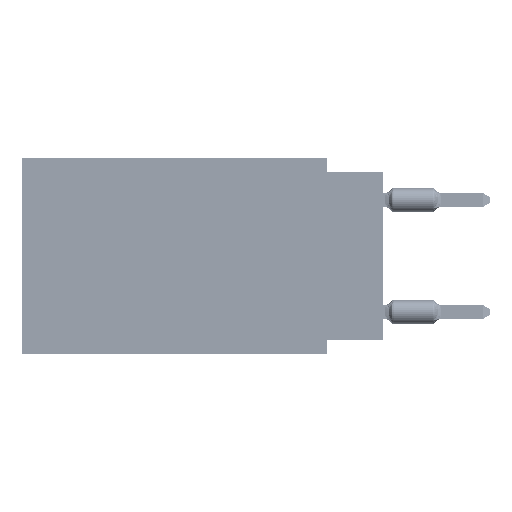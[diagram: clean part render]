
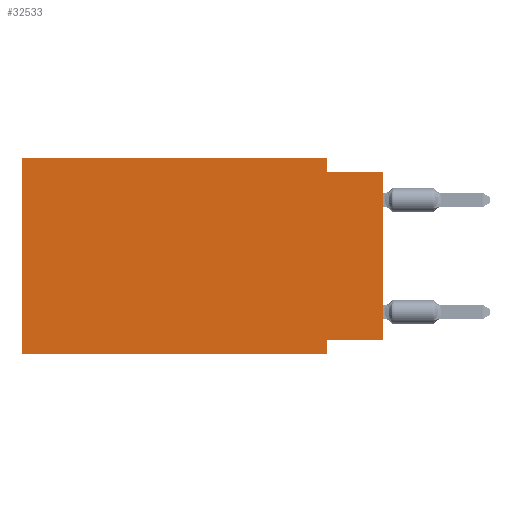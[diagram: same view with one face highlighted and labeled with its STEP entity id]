
A CAD part, left-side view. The second image highlights one B-rep face of the part: STEP entity #32533.
In plain terms, the highlighted planar face has unit normal (-1, 0, 0).
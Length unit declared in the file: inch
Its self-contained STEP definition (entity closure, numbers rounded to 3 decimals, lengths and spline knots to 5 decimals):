
#1469 = CARTESIAN_POINT ( 'NONE',  ( 0., 0., -0.025 ) ) ;
#1989 = EDGE_CURVE ( 'NONE', #17932, #36386, #73937, .T. ) ;
#2767 = CARTESIAN_POINT ( 'NONE',  ( 0., 0., -0.325 ) ) ;
#3506 = VERTEX_POINT ( 'NONE', #106104 ) ;
#4464 = DIRECTION ( 'NONE',  ( 0., 0., 1. ) ) ;
#6287 = ORIENTED_EDGE ( 'NONE', *, *, #96938, .T. ) ;
#7611 = CARTESIAN_POINT ( 'NONE',  ( 0., 0.1, -0.35 ) ) ;
#8929 = DIRECTION ( 'NONE',  ( 0., 0., -1. ) ) ;
#13136 = ORIENTED_EDGE ( 'NONE', *, *, #74413, .F. ) ;
#14028 = ORIENTED_EDGE ( 'NONE', *, *, #56712, .T. ) ;
#16276 = DIRECTION ( 'NONE',  ( 0., -1., 0. ) ) ;
#16744 = VECTOR ( 'NONE', #32953, 39.37008 ) ;
#17932 = VERTEX_POINT ( 'NONE', #60454 ) ;
#20745 = CARTESIAN_POINT ( 'NONE',  ( 0., 0., 0. ) ) ;
#21174 = CARTESIAN_POINT ( 'NONE',  ( 0., 0., -0.025 ) ) ;
#21676 = VERTEX_POINT ( 'NONE', #71001 ) ;
#21886 = DIRECTION ( 'NONE',  ( 0., 0., -1. ) ) ;
#26536 = VECTOR ( 'NONE', #16276, 39.37008 ) ;
#27663 = CARTESIAN_POINT ( 'NONE',  ( 0., 0.645, 0. ) ) ;
#29261 = LINE ( 'NONE', #21174, #70019 ) ;
#31399 = VERTEX_POINT ( 'NONE', #34176 ) ;
#32533 = ADVANCED_FACE ( 'NONE', ( #81167 ), #87672, .F. ) ;
#32953 = DIRECTION ( 'NONE',  ( 0., 0., -1. ) ) ;
#32995 = ORIENTED_EDGE ( 'NONE', *, *, #41083, .F. ) ;
#33418 = AXIS2_PLACEMENT_3D ( 'NONE', #56347, #55303, #21886 ) ;
#33515 = CARTESIAN_POINT ( 'NONE',  ( 0., 0.645, -0.35 ) ) ;
#34176 = CARTESIAN_POINT ( 'NONE',  ( 0., 0., -0.325 ) ) ;
#36386 = VERTEX_POINT ( 'NONE', #44296 ) ;
#36723 = LINE ( 'NONE', #2767, #80894 ) ;
#39363 = CARTESIAN_POINT ( 'NONE',  ( 0., 0.1, -0.025 ) ) ;
#40755 = CARTESIAN_POINT ( 'NONE',  ( 0., 0.1, 0. ) ) ;
#41083 = EDGE_CURVE ( 'NONE', #31399, #17932, #36723, .T. ) ;
#44296 = CARTESIAN_POINT ( 'NONE',  ( 0., 0.1, -0.35 ) ) ;
#44341 = LINE ( 'NONE', #27663, #56778 ) ;
#45364 = VECTOR ( 'NONE', #8929, 39.37008 ) ;
#49204 = LINE ( 'NONE', #82639, #53402 ) ;
#51661 = CARTESIAN_POINT ( 'NONE',  ( 0., 0.645, -0.35 ) ) ;
#51704 = VERTEX_POINT ( 'NONE', #39363 ) ;
#53402 = VECTOR ( 'NONE', #74020, 39.37008 ) ;
#53486 = VERTEX_POINT ( 'NONE', #1469 ) ;
#54056 = DIRECTION ( 'NONE',  ( 0., -1., 0. ) ) ;
#55303 = DIRECTION ( 'NONE',  ( 1., 0., 0. ) ) ;
#56347 = CARTESIAN_POINT ( 'NONE',  ( 0., 0.645, 0. ) ) ;
#56411 = LINE ( 'NONE', #40755, #45364 ) ;
#56712 = EDGE_CURVE ( 'NONE', #60900, #36386, #75028, .T. ) ;
#56778 = VECTOR ( 'NONE', #4464, 39.37008 ) ;
#60115 = EDGE_CURVE ( 'NONE', #51704, #53486, #29261, .T. ) ;
#60454 = CARTESIAN_POINT ( 'NONE',  ( 0., 0.1, -0.325 ) ) ;
#60900 = VERTEX_POINT ( 'NONE', #51661 ) ;
#67042 = ORIENTED_EDGE ( 'NONE', *, *, #84600, .F. ) ;
#70019 = VECTOR ( 'NONE', #54056, 39.37008 ) ;
#71001 = CARTESIAN_POINT ( 'NONE',  ( 0., 0.1, 0. ) ) ;
#73561 = VECTOR ( 'NONE', #81086, 39.37008 ) ;
#73937 = LINE ( 'NONE', #7611, #16744 ) ;
#74020 = DIRECTION ( 'NONE',  ( 0., -1., 0. ) ) ;
#74413 = EDGE_CURVE ( 'NONE', #60900, #3506, #44341, .T. ) ;
#75028 = LINE ( 'NONE', #33515, #26536 ) ;
#78824 = EDGE_CURVE ( 'NONE', #3506, #21676, #49204, .T. ) ;
#80894 = VECTOR ( 'NONE', #92820, 39.37008 ) ;
#81086 = DIRECTION ( 'NONE',  ( 0., 0., 1. ) ) ;
#81167 = FACE_OUTER_BOUND ( 'NONE', #96877, .T. ) ;
#82639 = CARTESIAN_POINT ( 'NONE',  ( 0., 0.645, 0. ) ) ;
#82845 = ORIENTED_EDGE ( 'NONE', *, *, #1989, .F. ) ;
#84600 = EDGE_CURVE ( 'NONE', #21676, #51704, #56411, .T. ) ;
#87672 = PLANE ( 'NONE',  #33418 ) ;
#92820 = DIRECTION ( 'NONE',  ( 0., 1., 0. ) ) ;
#96877 = EDGE_LOOP ( 'NONE', ( #6287, #103096, #67042, #97855, #13136, #14028, #82845, #32995 ) ) ;
#96938 = EDGE_CURVE ( 'NONE', #31399, #53486, #102706, .T. ) ;
#97855 = ORIENTED_EDGE ( 'NONE', *, *, #78824, .F. ) ;
#102706 = LINE ( 'NONE', #20745, #73561 ) ;
#103096 = ORIENTED_EDGE ( 'NONE', *, *, #60115, .F. ) ;
#106104 = CARTESIAN_POINT ( 'NONE',  ( 0., 0.645, 0. ) ) ;
